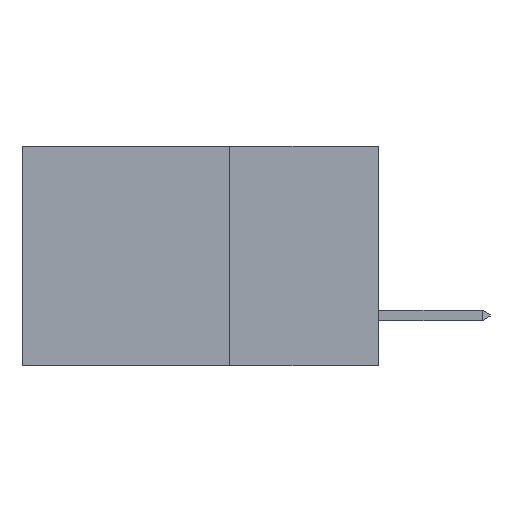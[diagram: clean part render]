
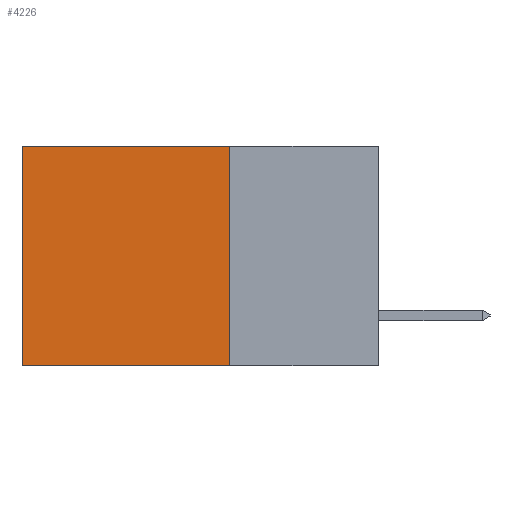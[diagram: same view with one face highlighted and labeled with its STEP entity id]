
A CAD part, left-side view. The second image highlights one B-rep face of the part: STEP entity #4226.
In plain terms, the highlighted planar face has unit normal (-1, 0, 0).
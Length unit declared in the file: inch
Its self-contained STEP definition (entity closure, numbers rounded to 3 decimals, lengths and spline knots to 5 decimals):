
#211 = CARTESIAN_POINT ( 'NONE',  ( 0.2615, 0.25, -0.37 ) ) ;
#417 = ORIENTED_EDGE ( 'NONE', *, *, #22695, .T. ) ;
#1490 = VERTEX_POINT ( 'NONE', #22930 ) ;
#1589 = VERTEX_POINT ( 'NONE', #21765 ) ;
#2225 = DIRECTION ( 'NONE',  ( 0., 0., -1. ) ) ;
#3089 = DIRECTION ( 'NONE',  ( 0., 1., 0. ) ) ;
#4226 = ADVANCED_FACE ( 'NONE', ( #18901 ), #6020, .F. ) ;
#5112 = DIRECTION ( 'NONE',  ( 0., 0., -1. ) ) ;
#5150 = DIRECTION ( 'NONE',  ( 1., 0., 0. ) ) ;
#5357 = CARTESIAN_POINT ( 'NONE',  ( 0.2615, 0.25, -0.37 ) ) ;
#6020 = PLANE ( 'NONE',  #23675 ) ;
#9001 = LINE ( 'NONE', #15213, #14393 ) ;
#10033 = ORIENTED_EDGE ( 'NONE', *, *, #14676, .T. ) ;
#10047 = ORIENTED_EDGE ( 'NONE', *, *, #22475, .F. ) ;
#11250 = LINE ( 'NONE', #211, #21356 ) ;
#11303 = VERTEX_POINT ( 'NONE', #17702 ) ;
#13818 = CARTESIAN_POINT ( 'NONE',  ( 0.2615, 0.6, -0.37 ) ) ;
#13996 = VECTOR ( 'NONE', #17367, 39.37008 ) ;
#14073 = LINE ( 'NONE', #13818, #24688 ) ;
#14393 = VECTOR ( 'NONE', #3089, 39.37008 ) ;
#14676 = EDGE_CURVE ( 'NONE', #19083, #1490, #25852, .T. ) ;
#15213 = CARTESIAN_POINT ( 'NONE',  ( 0.2615, 0.25, -0.37 ) ) ;
#15831 = DIRECTION ( 'NONE',  ( 0., 0., -1. ) ) ;
#16258 = EDGE_LOOP ( 'NONE', ( #417, #10047, #25200, #10033 ) ) ;
#17367 = DIRECTION ( 'NONE',  ( 0., 1., 0. ) ) ;
#17702 = CARTESIAN_POINT ( 'NONE',  ( 0.2615, 0.6, -0.37 ) ) ;
#18901 = FACE_OUTER_BOUND ( 'NONE', #16258, .T. ) ;
#19083 = VERTEX_POINT ( 'NONE', #20480 ) ;
#19382 = CARTESIAN_POINT ( 'NONE',  ( 0.2615, 0.25, 0. ) ) ;
#20480 = CARTESIAN_POINT ( 'NONE',  ( 0.2615, 0.25, 0. ) ) ;
#21356 = VECTOR ( 'NONE', #2225, 39.37008 ) ;
#21765 = CARTESIAN_POINT ( 'NONE',  ( 0.2615, 0.25, -0.37 ) ) ;
#22181 = EDGE_CURVE ( 'NONE', #19083, #1589, #11250, .T. ) ;
#22475 = EDGE_CURVE ( 'NONE', #1589, #11303, #9001, .T. ) ;
#22695 = EDGE_CURVE ( 'NONE', #1490, #11303, #14073, .T. ) ;
#22930 = CARTESIAN_POINT ( 'NONE',  ( 0.2615, 0.6, 0. ) ) ;
#23675 = AXIS2_PLACEMENT_3D ( 'NONE', #5357, #5150, #5112 ) ;
#24688 = VECTOR ( 'NONE', #15831, 39.37008 ) ;
#25200 = ORIENTED_EDGE ( 'NONE', *, *, #22181, .F. ) ;
#25852 = LINE ( 'NONE', #19382, #13996 ) ;
